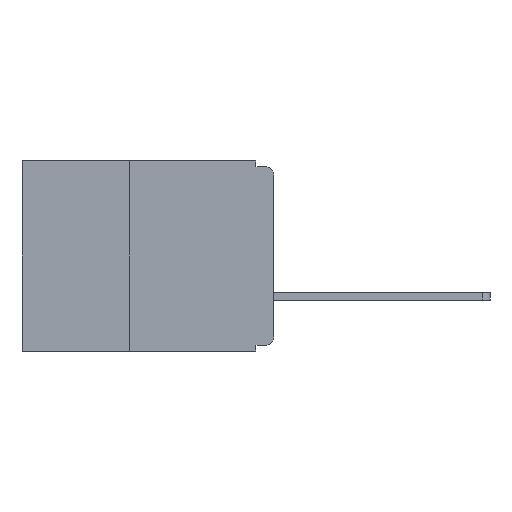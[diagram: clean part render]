
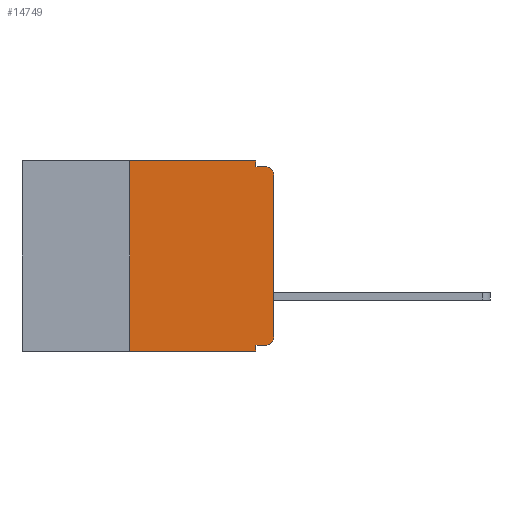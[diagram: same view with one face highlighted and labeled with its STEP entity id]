
A CAD part, left-side view. The second image highlights one B-rep face of the part: STEP entity #14749.
In plain terms, the highlighted planar face has unit normal (-1, 0, 0).
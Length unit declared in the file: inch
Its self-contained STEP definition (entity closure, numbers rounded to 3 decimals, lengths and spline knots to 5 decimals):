
#406 = EDGE_CURVE ( 'NONE', #7517, #15019, #10943, .T. ) ;
#607 = ORIENTED_EDGE ( 'NONE', *, *, #406, .F. ) ;
#932 = DIRECTION ( 'NONE',  ( 1., 0., 0. ) ) ;
#1092 = EDGE_CURVE ( 'NONE', #12644, #21905, #13191, .T. ) ;
#1770 = VECTOR ( 'NONE', #11979, 39.37008 ) ;
#2426 = CARTESIAN_POINT ( 'NONE',  ( 0., 0., -0.305 ) ) ;
#2453 = CARTESIAN_POINT ( 'NONE',  ( 0., 0.015, -0.025 ) ) ;
#2493 = LINE ( 'NONE', #25233, #1770 ) ;
#2776 = CARTESIAN_POINT ( 'NONE',  ( 0., 0.25, -0.33 ) ) ;
#3104 = CARTESIAN_POINT ( 'NONE',  ( 0., 0.437, 0. ) ) ;
#3211 = ORIENTED_EDGE ( 'NONE', *, *, #4227, .F. ) ;
#4184 = CARTESIAN_POINT ( 'NONE',  ( 0., 0.031, 0. ) ) ;
#4227 = EDGE_CURVE ( 'NONE', #15019, #21534, #18199, .T. ) ;
#4717 = VECTOR ( 'NONE', #10046, 39.37008 ) ;
#4755 = DIRECTION ( 'NONE',  ( 0., 0., -1. ) ) ;
#5322 = ORIENTED_EDGE ( 'NONE', *, *, #9751, .T. ) ;
#5676 = VECTOR ( 'NONE', #14687, 39.37008 ) ;
#5865 = VECTOR ( 'NONE', #15908, 39.37008 ) ;
#5960 = ORIENTED_EDGE ( 'NONE', *, *, #21373, .T. ) ;
#6458 = CARTESIAN_POINT ( 'NONE',  ( 0., 0.031, -0.33 ) ) ;
#6862 = EDGE_CURVE ( 'NONE', #21213, #7517, #28009, .T. ) ;
#7517 = VERTEX_POINT ( 'NONE', #25950 ) ;
#7738 = CARTESIAN_POINT ( 'NONE',  ( 0., 0.015, -0.305 ) ) ;
#8310 = CARTESIAN_POINT ( 'NONE',  ( 0., 0.031, -0.01 ) ) ;
#8585 = LINE ( 'NONE', #23376, #21123 ) ;
#8675 = CARTESIAN_POINT ( 'NONE',  ( 0., 0., -0.32 ) ) ;
#8739 = VERTEX_POINT ( 'NONE', #12643 ) ;
#9310 = VECTOR ( 'NONE', #10935, 39.37008 ) ;
#9751 = EDGE_CURVE ( 'NONE', #24451, #13812, #19306, .T. ) ;
#9988 = DIRECTION ( 'NONE',  ( 0., 0., -1. ) ) ;
#10046 = DIRECTION ( 'NONE',  ( 0., 0., 1. ) ) ;
#10935 = DIRECTION ( 'NONE',  ( 0., 1., 0. ) ) ;
#10943 = LINE ( 'NONE', #17361, #27845 ) ;
#11900 = CARTESIAN_POINT ( 'NONE',  ( 0., 0.031, -0.33 ) ) ;
#11979 = DIRECTION ( 'NONE',  ( 0., -1., 0. ) ) ;
#12316 = DIRECTION ( 'NONE',  ( 0., -1., 0. ) ) ;
#12643 = CARTESIAN_POINT ( 'NONE',  ( 0., 0.015, -0.32 ) ) ;
#12644 = VERTEX_POINT ( 'NONE', #26292 ) ;
#13191 = LINE ( 'NONE', #6458, #5865 ) ;
#13812 = VERTEX_POINT ( 'NONE', #22194 ) ;
#14047 = ORIENTED_EDGE ( 'NONE', *, *, #1092, .F. ) ;
#14324 = PLANE ( 'NONE',  #21390 ) ;
#14687 = DIRECTION ( 'NONE',  ( 0., 0., -1. ) ) ;
#14702 = EDGE_CURVE ( 'NONE', #21534, #13812, #2493, .T. ) ;
#14749 = ADVANCED_FACE ( 'NONE', ( #18185 ), #14324, .F. ) ;
#14780 = CARTESIAN_POINT ( 'NONE',  ( 0., 0.031, 0. ) ) ;
#15019 = VERTEX_POINT ( 'NONE', #4184 ) ;
#15908 = DIRECTION ( 'NONE',  ( 0., 0., -1. ) ) ;
#15924 = AXIS2_PLACEMENT_3D ( 'NONE', #2453, #18058, #4755 ) ;
#16329 = VECTOR ( 'NONE', #19263, 39.37008 ) ;
#16530 = DIRECTION ( 'NONE',  ( 0., 0., -1. ) ) ;
#17361 = CARTESIAN_POINT ( 'NONE',  ( 0., 0.437, 0. ) ) ;
#17443 = ORIENTED_EDGE ( 'NONE', *, *, #6862, .F. ) ;
#18005 = CIRCLE ( 'NONE', #18007, 0.015 ) ;
#18007 = AXIS2_PLACEMENT_3D ( 'NONE', #7738, #23278, #9988 ) ;
#18021 = EDGE_CURVE ( 'NONE', #8739, #12644, #26962, .T. ) ;
#18058 = DIRECTION ( 'NONE',  ( -1., 0., 0. ) ) ;
#18185 = FACE_OUTER_BOUND ( 'NONE', #19058, .T. ) ;
#18199 = LINE ( 'NONE', #14780, #5676 ) ;
#19058 = EDGE_LOOP ( 'NONE', ( #25506, #5322, #20960, #3211, #607, #17443, #21847, #14047, #22074, #5960 ) ) ;
#19263 = DIRECTION ( 'NONE',  ( 0., 0., 1. ) ) ;
#19292 = DIRECTION ( 'NONE',  ( 0., -1., 0. ) ) ;
#19306 = CIRCLE ( 'NONE', #15924, 0.015 ) ;
#20162 = CARTESIAN_POINT ( 'NONE',  ( 0., 0., -0.025 ) ) ;
#20960 = ORIENTED_EDGE ( 'NONE', *, *, #14702, .F. ) ;
#21123 = VECTOR ( 'NONE', #12316, 39.37008 ) ;
#21213 = VERTEX_POINT ( 'NONE', #2776 ) ;
#21373 = EDGE_CURVE ( 'NONE', #8739, #26793, #18005, .T. ) ;
#21390 = AXIS2_PLACEMENT_3D ( 'NONE', #3104, #932, #16530 ) ;
#21407 = EDGE_CURVE ( 'NONE', #21213, #21905, #8585, .T. ) ;
#21492 = CARTESIAN_POINT ( 'NONE',  ( 0., 0.25, -0.33 ) ) ;
#21534 = VERTEX_POINT ( 'NONE', #8310 ) ;
#21847 = ORIENTED_EDGE ( 'NONE', *, *, #21407, .T. ) ;
#21905 = VERTEX_POINT ( 'NONE', #11900 ) ;
#22074 = ORIENTED_EDGE ( 'NONE', *, *, #18021, .F. ) ;
#22194 = CARTESIAN_POINT ( 'NONE',  ( 0., 0.015, -0.01 ) ) ;
#22410 = LINE ( 'NONE', #25535, #4717 ) ;
#23278 = DIRECTION ( 'NONE',  ( -1., 0., 0. ) ) ;
#23376 = CARTESIAN_POINT ( 'NONE',  ( 0., 0.437, -0.33 ) ) ;
#24451 = VERTEX_POINT ( 'NONE', #20162 ) ;
#25233 = CARTESIAN_POINT ( 'NONE',  ( 0., 0., -0.01 ) ) ;
#25506 = ORIENTED_EDGE ( 'NONE', *, *, #28728, .T. ) ;
#25535 = CARTESIAN_POINT ( 'NONE',  ( 0., 0., 0. ) ) ;
#25950 = CARTESIAN_POINT ( 'NONE',  ( 0., 0.25, 0. ) ) ;
#26292 = CARTESIAN_POINT ( 'NONE',  ( 0., 0.031, -0.32 ) ) ;
#26793 = VERTEX_POINT ( 'NONE', #2426 ) ;
#26962 = LINE ( 'NONE', #8675, #9310 ) ;
#27845 = VECTOR ( 'NONE', #19292, 39.37008 ) ;
#28009 = LINE ( 'NONE', #21492, #16329 ) ;
#28728 = EDGE_CURVE ( 'NONE', #26793, #24451, #22410, .T. ) ;
